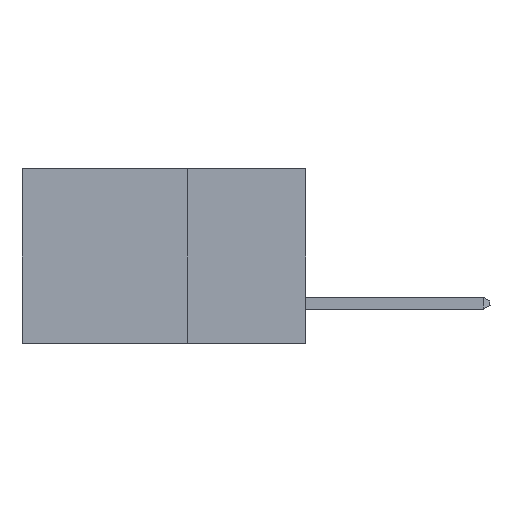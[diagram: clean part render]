
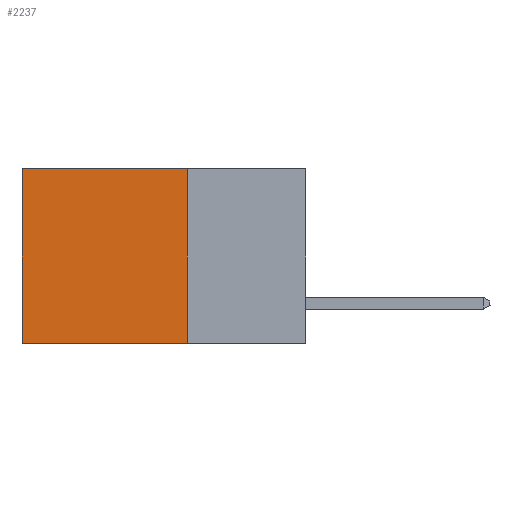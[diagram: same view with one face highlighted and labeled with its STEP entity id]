
A CAD part, left-side view. The second image highlights one B-rep face of the part: STEP entity #2237.
In plain terms, the highlighted planar face has unit normal (-1, 0, 0).
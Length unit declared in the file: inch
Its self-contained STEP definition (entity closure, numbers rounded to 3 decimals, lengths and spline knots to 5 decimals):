
#38 = PLANE ( 'NONE',  #1960 ) ;
#75 = VERTEX_POINT ( 'NONE', #4269 ) ;
#326 = LINE ( 'NONE', #8869, #8893 ) ;
#432 = VERTEX_POINT ( 'NONE', #9479 ) ;
#495 = FACE_OUTER_BOUND ( 'NONE', #6556, .T. ) ;
#876 = EDGE_CURVE ( 'NONE', #8904, #75, #8754, .T. ) ;
#1096 = DIRECTION ( 'NONE',  ( 1., 0., 0. ) ) ;
#1270 = ORIENTED_EDGE ( 'NONE', *, *, #3220, .T. ) ;
#1875 = ORIENTED_EDGE ( 'NONE', *, *, #2783, .F. ) ;
#1896 = DIRECTION ( 'NONE',  ( 0., 0., -1. ) ) ;
#1960 = AXIS2_PLACEMENT_3D ( 'NONE', #11009, #1096, #6598 ) ;
#2040 = VECTOR ( 'NONE', #12729, 39.37008 ) ;
#2237 = ADVANCED_FACE ( 'NONE', ( #495 ), #38, .F. ) ;
#2305 = CARTESIAN_POINT ( 'NONE',  ( 0.2615, 0.6, -0.37 ) ) ;
#2649 = CARTESIAN_POINT ( 'NONE',  ( 0.2615, 0.25, -0.37 ) ) ;
#2783 = EDGE_CURVE ( 'NONE', #432, #3560, #8362, .T. ) ;
#3220 = EDGE_CURVE ( 'NONE', #75, #3560, #13257, .T. ) ;
#3533 = ORIENTED_EDGE ( 'NONE', *, *, #5605, .F. ) ;
#3553 = VECTOR ( 'NONE', #13488, 39.37008 ) ;
#3560 = VERTEX_POINT ( 'NONE', #2305 ) ;
#4269 = CARTESIAN_POINT ( 'NONE',  ( 0.2615, 0.6, 0. ) ) ;
#5605 = EDGE_CURVE ( 'NONE', #8904, #432, #326, .T. ) ;
#6556 = EDGE_LOOP ( 'NONE', ( #1270, #1875, #3533, #8588 ) ) ;
#6598 = DIRECTION ( 'NONE',  ( 0., 0., -1. ) ) ;
#7319 = CARTESIAN_POINT ( 'NONE',  ( 0.2615, 0.6, -0.37 ) ) ;
#8362 = LINE ( 'NONE', #2649, #3553 ) ;
#8588 = ORIENTED_EDGE ( 'NONE', *, *, #876, .T. ) ;
#8754 = LINE ( 'NONE', #10538, #2040 ) ;
#8770 = DIRECTION ( 'NONE',  ( 0., 0., -1. ) ) ;
#8869 = CARTESIAN_POINT ( 'NONE',  ( 0.2615, 0.25, -0.37 ) ) ;
#8893 = VECTOR ( 'NONE', #8770, 39.37008 ) ;
#8904 = VERTEX_POINT ( 'NONE', #11553 ) ;
#9479 = CARTESIAN_POINT ( 'NONE',  ( 0.2615, 0.25, -0.37 ) ) ;
#10538 = CARTESIAN_POINT ( 'NONE',  ( 0.2615, 0.25, 0. ) ) ;
#11009 = CARTESIAN_POINT ( 'NONE',  ( 0.2615, 0.25, -0.37 ) ) ;
#11553 = CARTESIAN_POINT ( 'NONE',  ( 0.2615, 0.25, 0. ) ) ;
#12729 = DIRECTION ( 'NONE',  ( 0., 1., 0. ) ) ;
#13090 = VECTOR ( 'NONE', #1896, 39.37008 ) ;
#13257 = LINE ( 'NONE', #7319, #13090 ) ;
#13488 = DIRECTION ( 'NONE',  ( 0., 1., 0. ) ) ;
